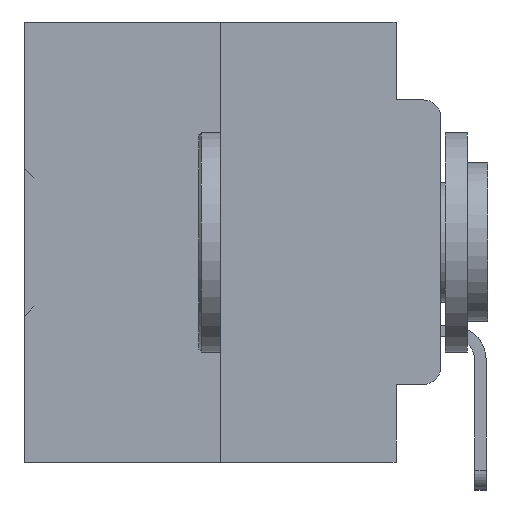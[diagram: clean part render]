
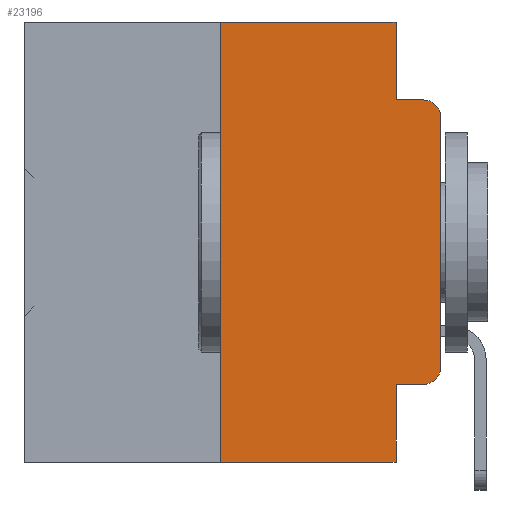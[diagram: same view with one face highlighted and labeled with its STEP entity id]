
A CAD part, left-side view. The second image highlights one B-rep face of the part: STEP entity #23196.
In plain terms, the highlighted planar face has unit normal (-1, 0, 0).
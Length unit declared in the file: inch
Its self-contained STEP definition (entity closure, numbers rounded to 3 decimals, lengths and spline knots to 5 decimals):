
#458 = DIRECTION ( 'NONE',  ( 0., -1., 0. ) ) ;
#979 = CARTESIAN_POINT ( 'NONE',  ( 0., 0.25, 0. ) ) ;
#1079 = AXIS2_PLACEMENT_3D ( 'NONE', #1630, #23107, #4861 ) ;
#1100 = VECTOR ( 'NONE', #458, 39.37008 ) ;
#1431 = DIRECTION ( 'NONE',  ( 0., -1., 0. ) ) ;
#1617 = CARTESIAN_POINT ( 'NONE',  ( 0., 0.02, -0.3915 ) ) ;
#1630 = CARTESIAN_POINT ( 'NONE',  ( 0., 0.02, -0.1085 ) ) ;
#1675 = VERTEX_POINT ( 'NONE', #17706 ) ;
#2140 = LINE ( 'NONE', #24402, #9542 ) ;
#3713 = CARTESIAN_POINT ( 'NONE',  ( 0., 0.051, -0.0885 ) ) ;
#4519 = DIRECTION ( 'NONE',  ( 0., 0., 1. ) ) ;
#4844 = DIRECTION ( 'NONE',  ( 0., 0., -1. ) ) ;
#4861 = DIRECTION ( 'NONE',  ( 0., 0., -1. ) ) ;
#5138 = CARTESIAN_POINT ( 'NONE',  ( 0., 0.473, 0. ) ) ;
#5166 = ORIENTED_EDGE ( 'NONE', *, *, #35091, .T. ) ;
#6055 = ORIENTED_EDGE ( 'NONE', *, *, #23425, .T. ) ;
#6871 = VERTEX_POINT ( 'NONE', #29378 ) ;
#8276 = CARTESIAN_POINT ( 'NONE',  ( 0., 0.051, -0.4115 ) ) ;
#8278 = DIRECTION ( 'NONE',  ( 0., 0., -1. ) ) ;
#8827 = ORIENTED_EDGE ( 'NONE', *, *, #27165, .F. ) ;
#9542 = VECTOR ( 'NONE', #21501, 39.37008 ) ;
#11116 = EDGE_CURVE ( 'NONE', #25341, #36202, #31601, .T. ) ;
#12366 = LINE ( 'NONE', #35176, #20374 ) ;
#12994 = VECTOR ( 'NONE', #17869, 39.37008 ) ;
#13147 = EDGE_CURVE ( 'NONE', #36202, #30125, #29103, .T. ) ;
#13229 = VERTEX_POINT ( 'NONE', #8276 ) ;
#14191 = EDGE_LOOP ( 'NONE', ( #38312, #29653, #24944, #8827, #16545, #19730, #6055, #32971, #5166, #34504 ) ) ;
#14409 = DIRECTION ( 'NONE',  ( 0., 0., -1. ) ) ;
#14918 = VERTEX_POINT ( 'NONE', #16577 ) ;
#15190 = AXIS2_PLACEMENT_3D ( 'NONE', #5138, #26366, #8278 ) ;
#16545 = ORIENTED_EDGE ( 'NONE', *, *, #37755, .F. ) ;
#16577 = CARTESIAN_POINT ( 'NONE',  ( 0., 0.051, -0.5 ) ) ;
#17210 = EDGE_CURVE ( 'NONE', #33356, #30125, #18577, .T. ) ;
#17706 = CARTESIAN_POINT ( 'NONE',  ( 0., 0.25, 0. ) ) ;
#17869 = DIRECTION ( 'NONE',  ( 0., 0., -1. ) ) ;
#17912 = LINE ( 'NONE', #22927, #23965 ) ;
#18140 = FACE_OUTER_BOUND ( 'NONE', #14191, .T. ) ;
#18577 = LINE ( 'NONE', #3713, #1100 ) ;
#18800 = CARTESIAN_POINT ( 'NONE',  ( 0., 0., -0.3915 ) ) ;
#19730 = ORIENTED_EDGE ( 'NONE', *, *, #29149, .F. ) ;
#20374 = VECTOR ( 'NONE', #14409, 39.37008 ) ;
#20378 = PLANE ( 'NONE',  #15190 ) ;
#20791 = VERTEX_POINT ( 'NONE', #34135 ) ;
#21501 = DIRECTION ( 'NONE',  ( 0., -1., 0. ) ) ;
#21830 = CARTESIAN_POINT ( 'NONE',  ( 0., 0., -0.1085 ) ) ;
#21893 = LINE ( 'NONE', #38574, #12994 ) ;
#22509 = DIRECTION ( 'NONE',  ( 0., 0., 1. ) ) ;
#22927 = CARTESIAN_POINT ( 'NONE',  ( 0., 0.051, -0.4115 ) ) ;
#23087 = DIRECTION ( 'NONE',  ( -1., 0., 0. ) ) ;
#23107 = DIRECTION ( 'NONE',  ( -1., 0., 0. ) ) ;
#23196 = ADVANCED_FACE ( 'NONE', ( #18140 ), #20378, .F. ) ;
#23425 = EDGE_CURVE ( 'NONE', #6871, #14918, #2140, .T. ) ;
#23471 = LINE ( 'NONE', #979, #30406 ) ;
#23676 = VERTEX_POINT ( 'NONE', #28382 ) ;
#23732 = VECTOR ( 'NONE', #4519, 39.37008 ) ;
#23849 = CARTESIAN_POINT ( 'NONE',  ( 0., 0.051, -0.0885 ) ) ;
#23965 = VECTOR ( 'NONE', #1431, 39.37008 ) ;
#24402 = CARTESIAN_POINT ( 'NONE',  ( 0., 0.473, -0.5 ) ) ;
#24944 = ORIENTED_EDGE ( 'NONE', *, *, #17210, .F. ) ;
#25341 = VERTEX_POINT ( 'NONE', #18800 ) ;
#26183 = CARTESIAN_POINT ( 'NONE',  ( 0., 0.473, 0. ) ) ;
#26366 = DIRECTION ( 'NONE',  ( 1., 0., 0. ) ) ;
#27165 = EDGE_CURVE ( 'NONE', #20791, #33356, #12366, .T. ) ;
#27373 = CARTESIAN_POINT ( 'NONE',  ( 0., 0.02, -0.0885 ) ) ;
#28382 = CARTESIAN_POINT ( 'NONE',  ( 0., 0.02, -0.4115 ) ) ;
#29103 = CIRCLE ( 'NONE', #1079, 0.02 ) ;
#29149 = EDGE_CURVE ( 'NONE', #6871, #1675, #23471, .T. ) ;
#29378 = CARTESIAN_POINT ( 'NONE',  ( 0., 0.25, -0.5 ) ) ;
#29653 = ORIENTED_EDGE ( 'NONE', *, *, #13147, .T. ) ;
#29747 = LINE ( 'NONE', #26183, #34837 ) ;
#30125 = VERTEX_POINT ( 'NONE', #27373 ) ;
#30406 = VECTOR ( 'NONE', #22509, 39.37008 ) ;
#31131 = EDGE_CURVE ( 'NONE', #13229, #14918, #21893, .T. ) ;
#31601 = LINE ( 'NONE', #34552, #23732 ) ;
#32971 = ORIENTED_EDGE ( 'NONE', *, *, #31131, .F. ) ;
#33356 = VERTEX_POINT ( 'NONE', #23849 ) ;
#34135 = CARTESIAN_POINT ( 'NONE',  ( 0., 0.051, 0. ) ) ;
#34504 = ORIENTED_EDGE ( 'NONE', *, *, #37075, .T. ) ;
#34552 = CARTESIAN_POINT ( 'NONE',  ( 0., 0., 0. ) ) ;
#34837 = VECTOR ( 'NONE', #35067, 39.37008 ) ;
#35067 = DIRECTION ( 'NONE',  ( 0., -1., 0. ) ) ;
#35091 = EDGE_CURVE ( 'NONE', #13229, #23676, #17912, .T. ) ;
#35176 = CARTESIAN_POINT ( 'NONE',  ( 0., 0.051, 0. ) ) ;
#36202 = VERTEX_POINT ( 'NONE', #21830 ) ;
#36266 = CIRCLE ( 'NONE', #38653, 0.02 ) ;
#37075 = EDGE_CURVE ( 'NONE', #23676, #25341, #36266, .T. ) ;
#37755 = EDGE_CURVE ( 'NONE', #1675, #20791, #29747, .T. ) ;
#38312 = ORIENTED_EDGE ( 'NONE', *, *, #11116, .T. ) ;
#38574 = CARTESIAN_POINT ( 'NONE',  ( 0., 0.051, 0. ) ) ;
#38653 = AXIS2_PLACEMENT_3D ( 'NONE', #1617, #23087, #4844 ) ;
